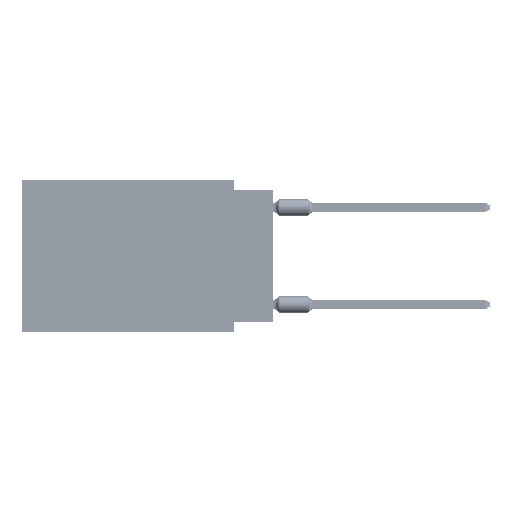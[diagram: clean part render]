
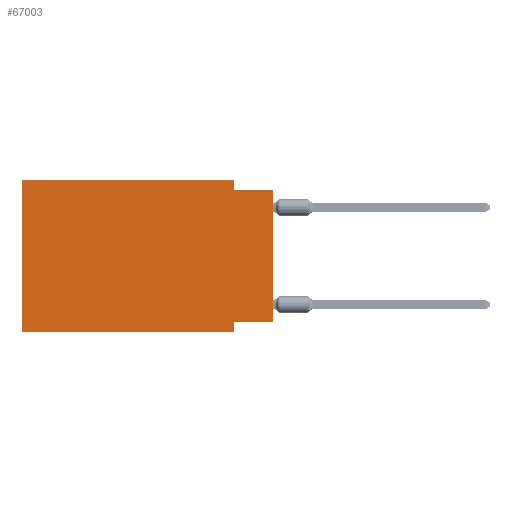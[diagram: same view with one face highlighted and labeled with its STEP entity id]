
A CAD part, left-side view. The second image highlights one B-rep face of the part: STEP entity #67003.
In plain terms, the highlighted planar face has unit normal (-1, 0, 0).
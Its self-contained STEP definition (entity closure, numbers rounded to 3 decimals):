
#407 = VERTEX_POINT ( 'NONE', #69099 ) ;
#1608 = DIRECTION ( 'NONE',  ( 0., 0., -1. ) ) ;
#1958 = CARTESIAN_POINT ( 'NONE',  ( 0., 16.383, 0. ) ) ;
#2566 = VECTOR ( 'NONE', #69553, 1000. ) ;
#2961 = VECTOR ( 'NONE', #52763, 1000. ) ;
#3788 = VERTEX_POINT ( 'NONE', #18864 ) ;
#4055 = ORIENTED_EDGE ( 'NONE', *, *, #9800, .F. ) ;
#7401 = DIRECTION ( 'NONE',  ( 1., 0., 0. ) ) ;
#8113 = CARTESIAN_POINT ( 'NONE',  ( 0., 16.383, 0. ) ) ;
#8483 = LINE ( 'NONE', #26297, #2566 ) ;
#8719 = EDGE_LOOP ( 'NONE', ( #46975, #71661, #55496, #55236, #62299, #40943, #4055, #48016 ) ) ;
#9800 = EDGE_CURVE ( 'NONE', #31126, #36681, #8483, .T. ) ;
#9945 = VERTEX_POINT ( 'NONE', #57293 ) ;
#11781 = DIRECTION ( 'NONE',  ( 0., 0., 1. ) ) ;
#12527 = VECTOR ( 'NONE', #19504, 1000. ) ;
#15425 = EDGE_CURVE ( 'NONE', #61036, #31126, #69861, .T. ) ;
#16350 = DIRECTION ( 'NONE',  ( 0., 0., 1. ) ) ;
#16753 = EDGE_CURVE ( 'NONE', #407, #36681, #64564, .T. ) ;
#17602 = LINE ( 'NONE', #1958, #33902 ) ;
#18864 = CARTESIAN_POINT ( 'NONE',  ( 0., 2.54, -0.635 ) ) ;
#18871 = CARTESIAN_POINT ( 'NONE',  ( 0., 2.54, 0. ) ) ;
#19504 = DIRECTION ( 'NONE',  ( 0., -1., 0. ) ) ;
#20574 = LINE ( 'NONE', #63839, #12527 ) ;
#23146 = LINE ( 'NONE', #8113, #49356 ) ;
#23186 = CARTESIAN_POINT ( 'NONE',  ( 0., 16.383, 0. ) ) ;
#26297 = CARTESIAN_POINT ( 'NONE',  ( 0., 2.54, -9.906 ) ) ;
#26402 = CARTESIAN_POINT ( 'NONE',  ( 0., 16.383, -9.906 ) ) ;
#27442 = VECTOR ( 'NONE', #42014, 1000. ) ;
#29937 = AXIS2_PLACEMENT_3D ( 'NONE', #57518, #7401, #1608 ) ;
#31126 = VERTEX_POINT ( 'NONE', #67694 ) ;
#33902 = VECTOR ( 'NONE', #11781, 1000. ) ;
#36681 = VERTEX_POINT ( 'NONE', #42136 ) ;
#37139 = CARTESIAN_POINT ( 'NONE',  ( 0., 0., -9.271 ) ) ;
#40943 = ORIENTED_EDGE ( 'NONE', *, *, #16753, .T. ) ;
#42014 = DIRECTION ( 'NONE',  ( 0., -1., 0. ) ) ;
#42136 = CARTESIAN_POINT ( 'NONE',  ( 0., 2.54, -9.906 ) ) ;
#43780 = EDGE_CURVE ( 'NONE', #407, #70859, #17602, .T. ) ;
#46968 = PLANE ( 'NONE',  #29937 ) ;
#46975 = ORIENTED_EDGE ( 'NONE', *, *, #62984, .T. ) ;
#48016 = ORIENTED_EDGE ( 'NONE', *, *, #15425, .F. ) ;
#49356 = VECTOR ( 'NONE', #50380, 1000. ) ;
#49382 = CARTESIAN_POINT ( 'NONE',  ( 0., 0., 0. ) ) ;
#50380 = DIRECTION ( 'NONE',  ( 0., -1., 0. ) ) ;
#50601 = CARTESIAN_POINT ( 'NONE',  ( 0., 0., -9.271 ) ) ;
#51709 = EDGE_CURVE ( 'NONE', #70859, #9945, #23146, .T. ) ;
#52534 = EDGE_CURVE ( 'NONE', #9945, #3788, #68647, .T. ) ;
#52763 = DIRECTION ( 'NONE',  ( 0., 1., 0. ) ) ;
#54357 = EDGE_CURVE ( 'NONE', #3788, #59745, #20574, .T. ) ;
#55236 = ORIENTED_EDGE ( 'NONE', *, *, #51709, .F. ) ;
#55496 = ORIENTED_EDGE ( 'NONE', *, *, #52534, .F. ) ;
#57293 = CARTESIAN_POINT ( 'NONE',  ( 0., 2.54, 0. ) ) ;
#57518 = CARTESIAN_POINT ( 'NONE',  ( 0., 16.383, 0. ) ) ;
#58393 = VECTOR ( 'NONE', #16350, 1000. ) ;
#59745 = VERTEX_POINT ( 'NONE', #66545 ) ;
#61036 = VERTEX_POINT ( 'NONE', #50601 ) ;
#62299 = ORIENTED_EDGE ( 'NONE', *, *, #43780, .F. ) ;
#62984 = EDGE_CURVE ( 'NONE', #61036, #59745, #66125, .T. ) ;
#63839 = CARTESIAN_POINT ( 'NONE',  ( 0., 0., -0.635 ) ) ;
#64564 = LINE ( 'NONE', #26402, #27442 ) ;
#66125 = LINE ( 'NONE', #49382, #58393 ) ;
#66545 = CARTESIAN_POINT ( 'NONE',  ( 0., 0., -0.635 ) ) ;
#67003 = ADVANCED_FACE ( 'NONE', ( #68098 ), #46968, .F. ) ;
#67575 = DIRECTION ( 'NONE',  ( 0., 0., -1. ) ) ;
#67694 = CARTESIAN_POINT ( 'NONE',  ( 0., 2.54, -9.271 ) ) ;
#68098 = FACE_OUTER_BOUND ( 'NONE', #8719, .T. ) ;
#68647 = LINE ( 'NONE', #18871, #70382 ) ;
#69099 = CARTESIAN_POINT ( 'NONE',  ( 0., 16.383, -9.906 ) ) ;
#69553 = DIRECTION ( 'NONE',  ( 0., 0., -1. ) ) ;
#69861 = LINE ( 'NONE', #37139, #2961 ) ;
#70382 = VECTOR ( 'NONE', #67575, 1000. ) ;
#70859 = VERTEX_POINT ( 'NONE', #23186 ) ;
#71661 = ORIENTED_EDGE ( 'NONE', *, *, #54357, .F. ) ;
